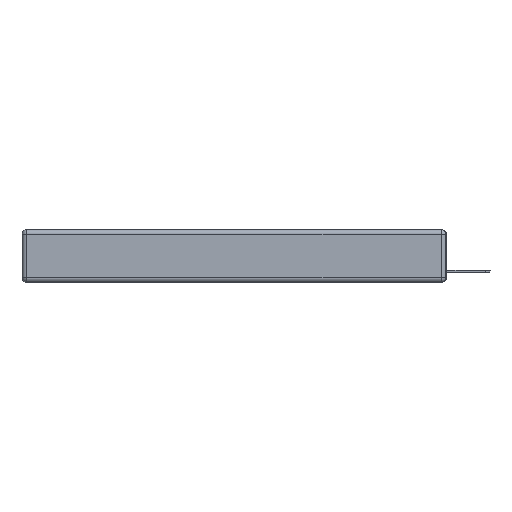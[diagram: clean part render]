
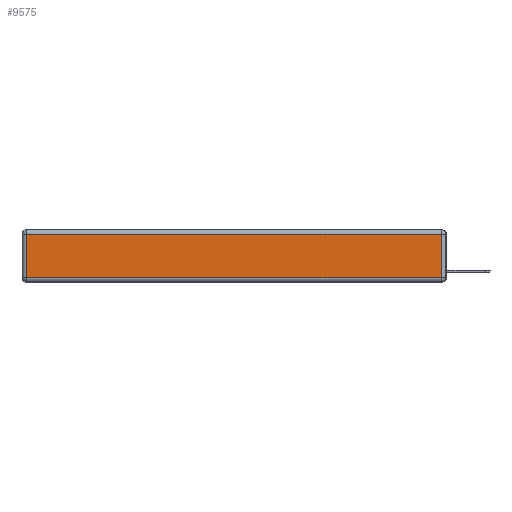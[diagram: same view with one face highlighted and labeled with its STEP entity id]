
A CAD part, left-side view. The second image highlights one B-rep face of the part: STEP entity #9575.
In plain terms, the highlighted planar face has unit normal (-1, 0, 0).
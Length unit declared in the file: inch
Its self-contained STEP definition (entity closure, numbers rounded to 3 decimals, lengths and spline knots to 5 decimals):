
#10 = CARTESIAN_POINT ( 'NONE',  ( 0., 0.03, -0.313 ) ) ;
#691 = VECTOR ( 'NONE', #2622, 39.37008 ) ;
#953 = ORIENTED_EDGE ( 'NONE', *, *, #14873, .T. ) ;
#994 = PLANE ( 'NONE',  #2361 ) ;
#1529 = CARTESIAN_POINT ( 'NONE',  ( 0., 0.03, -0.343 ) ) ;
#1634 = LINE ( 'NONE', #11850, #11015 ) ;
#2177 = EDGE_LOOP ( 'NONE', ( #4202, #4517, #8791, #953 ) ) ;
#2361 = AXIS2_PLACEMENT_3D ( 'NONE', #4656, #10308, #6834 ) ;
#2622 = DIRECTION ( 'NONE',  ( 0., 0., 1. ) ) ;
#2709 = VERTEX_POINT ( 'NONE', #11396 ) ;
#2721 = VERTEX_POINT ( 'NONE', #6295 ) ;
#3628 = LINE ( 'NONE', #1529, #691 ) ;
#3689 = FACE_OUTER_BOUND ( 'NONE', #2177, .T. ) ;
#4133 = EDGE_CURVE ( 'NONE', #15152, #2709, #1634, .T. ) ;
#4202 = ORIENTED_EDGE ( 'NONE', *, *, #13847, .T. ) ;
#4517 = ORIENTED_EDGE ( 'NONE', *, *, #4919, .T. ) ;
#4656 = CARTESIAN_POINT ( 'NONE',  ( 0., 0., -0.343 ) ) ;
#4919 = EDGE_CURVE ( 'NONE', #5099, #15152, #3628, .T. ) ;
#5025 = VECTOR ( 'NONE', #9114, 39.37008 ) ;
#5099 = VERTEX_POINT ( 'NONE', #10 ) ;
#5208 = DIRECTION ( 'NONE',  ( 0., -1., 0. ) ) ;
#6295 = CARTESIAN_POINT ( 'NONE',  ( 0., 2.72, -0.313 ) ) ;
#6834 = DIRECTION ( 'NONE',  ( 0., 0., 1. ) ) ;
#7273 = VECTOR ( 'NONE', #5208, 39.37008 ) ;
#8152 = LINE ( 'NONE', #15098, #5025 ) ;
#8791 = ORIENTED_EDGE ( 'NONE', *, *, #4133, .T. ) ;
#9114 = DIRECTION ( 'NONE',  ( 0., 0., -1. ) ) ;
#9575 = ADVANCED_FACE ( 'NONE', ( #3689 ), #994, .T. ) ;
#9596 = CARTESIAN_POINT ( 'NONE',  ( 0., 0.03, -0.03 ) ) ;
#9650 = LINE ( 'NONE', #12252, #7273 ) ;
#10308 = DIRECTION ( 'NONE',  ( -1., 0., 0. ) ) ;
#11015 = VECTOR ( 'NONE', #11797, 39.37008 ) ;
#11396 = CARTESIAN_POINT ( 'NONE',  ( 0., 2.72, -0.03 ) ) ;
#11797 = DIRECTION ( 'NONE',  ( 0., 1., 0. ) ) ;
#11850 = CARTESIAN_POINT ( 'NONE',  ( 0., 2.75, -0.03 ) ) ;
#12252 = CARTESIAN_POINT ( 'NONE',  ( 0., 0., -0.313 ) ) ;
#13847 = EDGE_CURVE ( 'NONE', #2721, #5099, #9650, .T. ) ;
#14873 = EDGE_CURVE ( 'NONE', #2709, #2721, #8152, .T. ) ;
#15098 = CARTESIAN_POINT ( 'NONE',  ( 0., 2.72, -0.343 ) ) ;
#15152 = VERTEX_POINT ( 'NONE', #9596 ) ;
